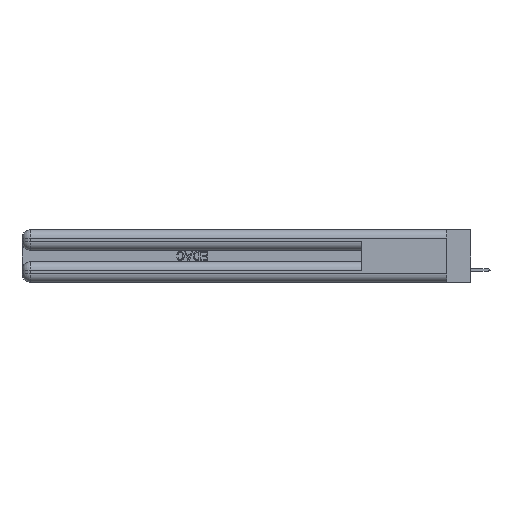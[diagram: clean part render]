
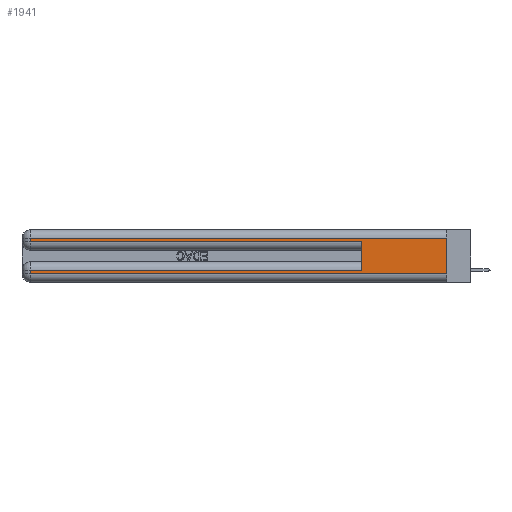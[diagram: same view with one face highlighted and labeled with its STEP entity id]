
A CAD part, left-side view. The second image highlights one B-rep face of the part: STEP entity #1941.
In plain terms, the highlighted planar face has unit normal (-1, 0, 0).
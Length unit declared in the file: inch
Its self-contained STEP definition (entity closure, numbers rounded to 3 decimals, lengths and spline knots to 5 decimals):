
#1941 = ADVANCED_FACE ( 'NONE', ( #7689 ), #27527, .F. ) ;
#2449 = LINE ( 'NONE', #5588, #2702 ) ;
#2702 = VECTOR ( 'NONE', #35018, 39.37008 ) ;
#5588 = CARTESIAN_POINT ( 'NONE',  ( 0., 2.94, 0.37 ) ) ;
#7048 = ORIENTED_EDGE ( 'NONE', *, *, #33451, .F. ) ;
#7689 = FACE_OUTER_BOUND ( 'NONE', #8575, .T. ) ;
#8575 = EDGE_LOOP ( 'NONE', ( #7048, #19391, #8616, #9110, #22287, #30406, #35966, #23990 ) ) ;
#8616 = ORIENTED_EDGE ( 'NONE', *, *, #14600, .T. ) ;
#9110 = ORIENTED_EDGE ( 'NONE', *, *, #25203, .T. ) ;
#9219 = VERTEX_POINT ( 'NONE', #21955 ) ;
#9241 = VERTEX_POINT ( 'NONE', #31801 ) ;
#10418 = DIRECTION ( 'NONE',  ( 0., 0., -1. ) ) ;
#11362 = DIRECTION ( 'NONE',  ( 0., 1., 0. ) ) ;
#11383 = CARTESIAN_POINT ( 'NONE',  ( 0., 2.94, 0.06 ) ) ;
#12347 = DIRECTION ( 'NONE',  ( 0., 1., 0. ) ) ;
#12626 = EDGE_CURVE ( 'NONE', #16659, #17637, #28031, .T. ) ;
#14600 = EDGE_CURVE ( 'NONE', #17637, #33694, #2449, .T. ) ;
#15085 = LINE ( 'NONE', #40161, #28059 ) ;
#16659 = VERTEX_POINT ( 'NONE', #25139 ) ;
#16876 = CARTESIAN_POINT ( 'NONE',  ( 0., 2.94, 0.31 ) ) ;
#17637 = VERTEX_POINT ( 'NONE', #16876 ) ;
#19389 = EDGE_CURVE ( 'NONE', #40927, #9219, #29570, .T. ) ;
#19391 = ORIENTED_EDGE ( 'NONE', *, *, #12626, .T. ) ;
#19553 = CARTESIAN_POINT ( 'NONE',  ( 0., 0., 0.06 ) ) ;
#19673 = VECTOR ( 'NONE', #20153, 39.37008 ) ;
#19890 = VECTOR ( 'NONE', #10418, 39.37008 ) ;
#19914 = EDGE_CURVE ( 'NONE', #31170, #33897, #33904, .T. ) ;
#20153 = DIRECTION ( 'NONE',  ( 0., -1., 0. ) ) ;
#20810 = DIRECTION ( 'NONE',  ( 0., 0., -1. ) ) ;
#21360 = LINE ( 'NONE', #28474, #35916 ) ;
#21955 = CARTESIAN_POINT ( 'NONE',  ( 0., 0., 0.06 ) ) ;
#22287 = ORIENTED_EDGE ( 'NONE', *, *, #19914, .F. ) ;
#23754 = CARTESIAN_POINT ( 'NONE',  ( 0., 0., 0.37 ) ) ;
#23990 = ORIENTED_EDGE ( 'NONE', *, *, #19389, .T. ) ;
#24878 = VECTOR ( 'NONE', #12347, 39.37008 ) ;
#25139 = CARTESIAN_POINT ( 'NONE',  ( 0., 0., 0.31 ) ) ;
#25203 = EDGE_CURVE ( 'NONE', #33694, #33897, #21360, .T. ) ;
#25467 = LINE ( 'NONE', #32747, #19890 ) ;
#26738 = VECTOR ( 'NONE', #37471, 39.37008 ) ;
#27527 = PLANE ( 'NONE',  #27627 ) ;
#27627 = AXIS2_PLACEMENT_3D ( 'NONE', #23754, #40262, #20810 ) ;
#28031 = LINE ( 'NONE', #31368, #24878 ) ;
#28059 = VECTOR ( 'NONE', #11362, 39.37008 ) ;
#28474 = CARTESIAN_POINT ( 'NONE',  ( 0., 0., 0.285 ) ) ;
#28839 = EDGE_CURVE ( 'NONE', #9241, #40927, #25467, .T. ) ;
#29570 = LINE ( 'NONE', #19553, #19673 ) ;
#29932 = DIRECTION ( 'NONE',  ( 0., 0., 1. ) ) ;
#30380 = LINE ( 'NONE', #33511, #26738 ) ;
#30406 = ORIENTED_EDGE ( 'NONE', *, *, #33791, .T. ) ;
#31170 = VERTEX_POINT ( 'NONE', #36882 ) ;
#31368 = CARTESIAN_POINT ( 'NONE',  ( 0., 0., 0.31 ) ) ;
#31801 = CARTESIAN_POINT ( 'NONE',  ( 0., 2.94, 0.085 ) ) ;
#32747 = CARTESIAN_POINT ( 'NONE',  ( 0., 2.94, 0.37 ) ) ;
#32857 = CARTESIAN_POINT ( 'NONE',  ( 0., 2.94, 0.285 ) ) ;
#33451 = EDGE_CURVE ( 'NONE', #16659, #9219, #30380, .T. ) ;
#33466 = CARTESIAN_POINT ( 'NONE',  ( 0., 0.6, 0.285 ) ) ;
#33511 = CARTESIAN_POINT ( 'NONE',  ( 0., 0., 0.37 ) ) ;
#33694 = VERTEX_POINT ( 'NONE', #32857 ) ;
#33791 = EDGE_CURVE ( 'NONE', #31170, #9241, #15085, .T. ) ;
#33897 = VERTEX_POINT ( 'NONE', #33466 ) ;
#33904 = LINE ( 'NONE', #36826, #41050 ) ;
#35018 = DIRECTION ( 'NONE',  ( 0., 0., -1. ) ) ;
#35916 = VECTOR ( 'NONE', #41001, 39.37008 ) ;
#35966 = ORIENTED_EDGE ( 'NONE', *, *, #28839, .T. ) ;
#36826 = CARTESIAN_POINT ( 'NONE',  ( 0., 0.6, 0.145 ) ) ;
#36882 = CARTESIAN_POINT ( 'NONE',  ( 0., 0.6, 0.085 ) ) ;
#37471 = DIRECTION ( 'NONE',  ( 0., 0., -1. ) ) ;
#40161 = CARTESIAN_POINT ( 'NONE',  ( 0., 0., 0.085 ) ) ;
#40262 = DIRECTION ( 'NONE',  ( 1., 0., 0. ) ) ;
#40927 = VERTEX_POINT ( 'NONE', #11383 ) ;
#41001 = DIRECTION ( 'NONE',  ( 0., -1., 0. ) ) ;
#41050 = VECTOR ( 'NONE', #29932, 39.37008 ) ;
